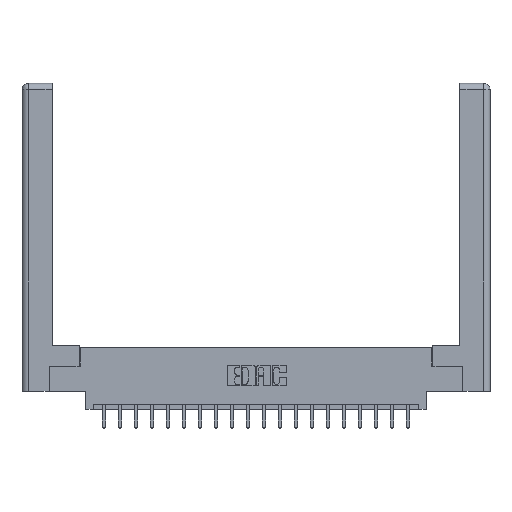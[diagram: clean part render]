
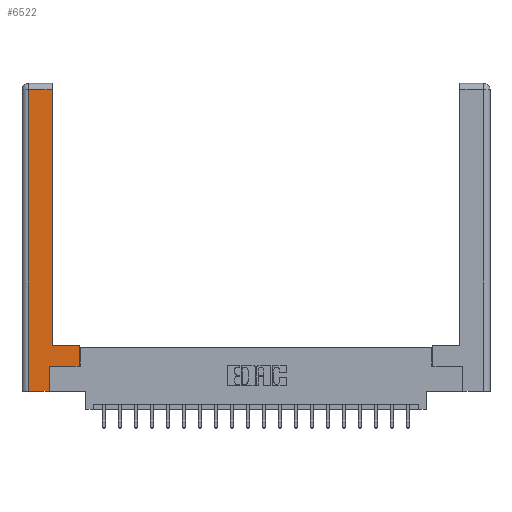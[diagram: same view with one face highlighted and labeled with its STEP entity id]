
A CAD part, top view. The second image highlights one B-rep face of the part: STEP entity #6522.
In plain terms, the highlighted planar face has unit normal (0, 0, 1).
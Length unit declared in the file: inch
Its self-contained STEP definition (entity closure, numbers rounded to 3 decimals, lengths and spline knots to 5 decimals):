
#131 = CARTESIAN_POINT ( 'NONE',  ( 0.0615, 0., 0. ) ) ;
#167 = LINE ( 'NONE', #3536, #16562 ) ;
#1244 = VECTOR ( 'NONE', #19977, 39.37008 ) ;
#1327 = CARTESIAN_POINT ( 'NONE',  ( 0.265, 0., 0. ) ) ;
#2034 = VECTOR ( 'NONE', #20359, 39.37008 ) ;
#2467 = LINE ( 'NONE', #14288, #8635 ) ;
#2508 = CARTESIAN_POINT ( 'NONE',  ( 0.565, 0.45, 0. ) ) ;
#2654 = DIRECTION ( 'NONE',  ( 0., 1., 0. ) ) ;
#2785 = LINE ( 'NONE', #131, #1244 ) ;
#2790 = CARTESIAN_POINT ( 'NONE',  ( 0.0615, 0., 0. ) ) ;
#3199 = CARTESIAN_POINT ( 'NONE',  ( 0., 0., 0. ) ) ;
#3392 = CARTESIAN_POINT ( 'NONE',  ( 0.565, 0.245, 0. ) ) ;
#3536 = CARTESIAN_POINT ( 'NONE',  ( 0.295, 0.45, 0. ) ) ;
#3798 = LINE ( 'NONE', #5891, #11236 ) ;
#3948 = ORIENTED_EDGE ( 'NONE', *, *, #16732, .T. ) ;
#4095 = DIRECTION ( 'NONE',  ( 0., 1., 0. ) ) ;
#4206 = VERTEX_POINT ( 'NONE', #3392 ) ;
#5244 = VECTOR ( 'NONE', #2654, 39.37008 ) ;
#5745 = LINE ( 'NONE', #2508, #5244 ) ;
#5825 = LINE ( 'NONE', #12231, #2034 ) ;
#5891 = CARTESIAN_POINT ( 'NONE',  ( 0.565, 0.245, 0. ) ) ;
#5918 = AXIS2_PLACEMENT_3D ( 'NONE', #3199, #14698, #16313 ) ;
#6330 = EDGE_CURVE ( 'NONE', #19081, #16927, #9251, .T. ) ;
#6522 = ADVANCED_FACE ( 'NONE', ( #15141 ), #9800, .F. ) ;
#8216 = LINE ( 'NONE', #18811, #16140 ) ;
#8346 = VERTEX_POINT ( 'NONE', #16311 ) ;
#8627 = ORIENTED_EDGE ( 'NONE', *, *, #9462, .T. ) ;
#8634 = EDGE_CURVE ( 'NONE', #4206, #8868, #5745, .T. ) ;
#8635 = VECTOR ( 'NONE', #12682, 39.37008 ) ;
#8835 = VERTEX_POINT ( 'NONE', #2790 ) ;
#8868 = VERTEX_POINT ( 'NONE', #9826 ) ;
#9251 = LINE ( 'NONE', #14269, #20277 ) ;
#9462 = EDGE_CURVE ( 'NONE', #8868, #8346, #167, .T. ) ;
#9800 = PLANE ( 'NONE',  #5918 ) ;
#9826 = CARTESIAN_POINT ( 'NONE',  ( 0.565, 0.45, 0. ) ) ;
#9873 = ORIENTED_EDGE ( 'NONE', *, *, #15259, .T. ) ;
#10733 = CARTESIAN_POINT ( 'NONE',  ( 0.265, 0.245, 0. ) ) ;
#11236 = VECTOR ( 'NONE', #19188, 39.37008 ) ;
#11658 = VERTEX_POINT ( 'NONE', #1327 ) ;
#12087 = EDGE_LOOP ( 'NONE', ( #15804, #15632, #9873, #12603, #3948, #18769, #19625, #8627 ) ) ;
#12231 = CARTESIAN_POINT ( 'NONE',  ( 0.265, 0., 0. ) ) ;
#12266 = CARTESIAN_POINT ( 'NONE',  ( 0.0615, 2.94, 0. ) ) ;
#12603 = ORIENTED_EDGE ( 'NONE', *, *, #20179, .T. ) ;
#12682 = DIRECTION ( 'NONE',  ( 0., 1., 0. ) ) ;
#14269 = CARTESIAN_POINT ( 'NONE',  ( 0.0615, 2.94, 0. ) ) ;
#14288 = CARTESIAN_POINT ( 'NONE',  ( 0.265, 0.245, 0. ) ) ;
#14698 = DIRECTION ( 'NONE',  ( 0., 0., -1. ) ) ;
#15022 = EDGE_CURVE ( 'NONE', #20263, #4206, #3798, .T. ) ;
#15141 = FACE_OUTER_BOUND ( 'NONE', #12087, .T. ) ;
#15259 = EDGE_CURVE ( 'NONE', #16927, #8835, #2785, .T. ) ;
#15632 = ORIENTED_EDGE ( 'NONE', *, *, #6330, .T. ) ;
#15804 = ORIENTED_EDGE ( 'NONE', *, *, #19800, .T. ) ;
#16131 = DIRECTION ( 'NONE',  ( -1., 0., 0. ) ) ;
#16140 = VECTOR ( 'NONE', #4095, 39.37008 ) ;
#16311 = CARTESIAN_POINT ( 'NONE',  ( 0.295, 0.45, 0. ) ) ;
#16313 = DIRECTION ( 'NONE',  ( -1., 0., 0. ) ) ;
#16562 = VECTOR ( 'NONE', #16131, 39.37008 ) ;
#16732 = EDGE_CURVE ( 'NONE', #11658, #20263, #2467, .T. ) ;
#16927 = VERTEX_POINT ( 'NONE', #12266 ) ;
#17515 = CARTESIAN_POINT ( 'NONE',  ( 0.295, 2.94, 0. ) ) ;
#18769 = ORIENTED_EDGE ( 'NONE', *, *, #15022, .T. ) ;
#18811 = CARTESIAN_POINT ( 'NONE',  ( 0.295, 3., 0. ) ) ;
#19081 = VERTEX_POINT ( 'NONE', #17515 ) ;
#19188 = DIRECTION ( 'NONE',  ( 1., 0., 0. ) ) ;
#19625 = ORIENTED_EDGE ( 'NONE', *, *, #8634, .T. ) ;
#19800 = EDGE_CURVE ( 'NONE', #8346, #19081, #8216, .T. ) ;
#19977 = DIRECTION ( 'NONE',  ( 0., -1., 0. ) ) ;
#20179 = EDGE_CURVE ( 'NONE', #8835, #11658, #5825, .T. ) ;
#20263 = VERTEX_POINT ( 'NONE', #10733 ) ;
#20277 = VECTOR ( 'NONE', #21067, 39.37008 ) ;
#20359 = DIRECTION ( 'NONE',  ( 1., 0., 0. ) ) ;
#21067 = DIRECTION ( 'NONE',  ( -1., 0., 0. ) ) ;
